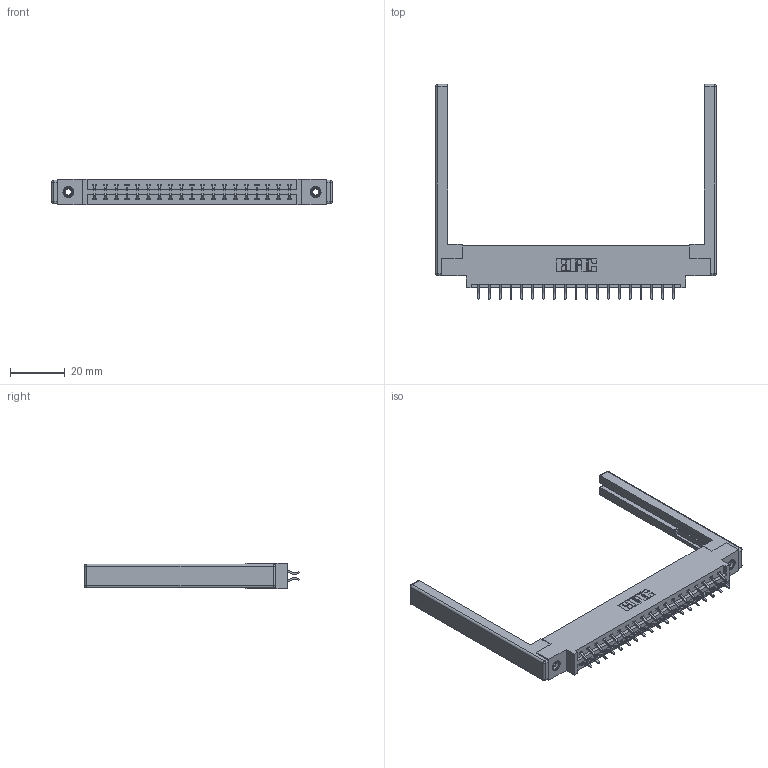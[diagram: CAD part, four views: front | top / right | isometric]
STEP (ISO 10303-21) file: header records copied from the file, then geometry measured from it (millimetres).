
FILE_DESCRIPTION (( 'STEP AP203' ), '1' );
FILE_NAME ('387-038-556-868.STEP', '2019-10-17T22:19:31', ( '' ), ( '' ), 'SwSTEP 2.0', 'SolidWorks 2016', '' );
FILE_SCHEMA (( 'CONFIG_CONTROL_DESIGN' ));
Length unit declared in the file: inch
Products named in the file (5): 345-250-001_345-250-001-102; 345-292-001_556 Tail; 307-220-068; 387-038-556-868; 337 Part_0.170 Offset - 0.156 Dia-TI
Assembly tree (43 placements, depth 2):
  387-038-556-868
    337 Part_0.170 Offset - 0.156 Dia-TI
    345-292-001_556 Tail  x38
    345-250-001_345-250-001-102  x2
    307-220-068  x2
Bounding box: 102.72 x 78.63 x 9.4 mm (x, y, z)
Volume: 14784.8 mm3; surface area: 15635.9 mm2
Topology: 43 solids, 43 shells, 2552 faces, 7515 edges, 4938 vertices
Faces by surface type: plane 1758, cylinder 770, cone 12, sphere 8, torus 4
Entity records: 20818 total; most frequent: CARTESIAN_POINT 3507, ORIENTED_EDGE 3420, DIRECTION 3084, EDGE_CURVE 1710, LINE 1524, VECTOR 1524, VERTEX_POINT 1130, AXIS2_PLACEMENT_3D 780
